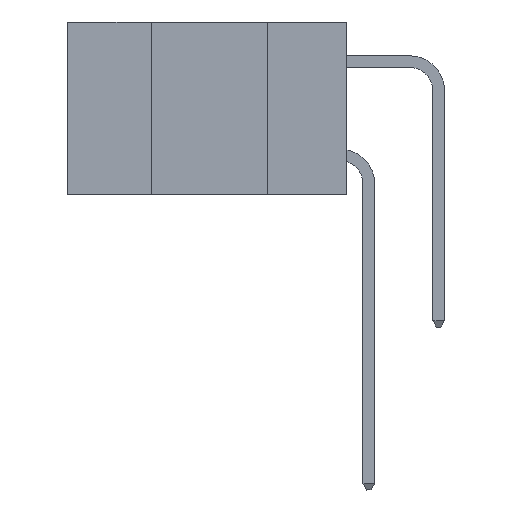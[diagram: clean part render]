
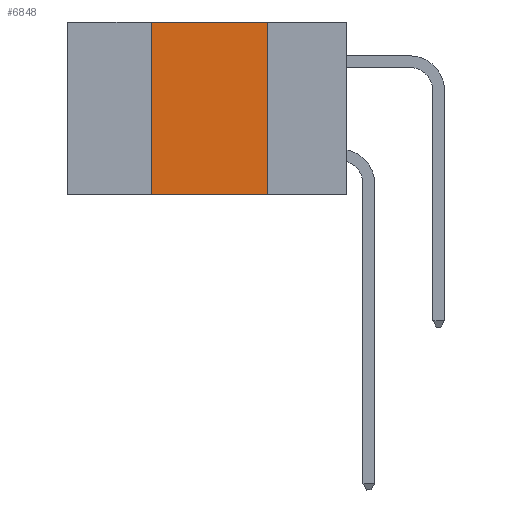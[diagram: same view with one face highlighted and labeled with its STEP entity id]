
A CAD part, left-side view. The second image highlights one B-rep face of the part: STEP entity #6848.
In plain terms, the highlighted planar face has unit normal (-1, 0, 0).
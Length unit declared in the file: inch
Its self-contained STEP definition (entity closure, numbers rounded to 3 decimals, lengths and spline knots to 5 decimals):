
#273 = VECTOR ( 'NONE', #11545, 39.37008 ) ;
#1991 = DIRECTION ( 'NONE',  ( 0., 0., -1. ) ) ;
#3389 = VECTOR ( 'NONE', #14678, 39.37008 ) ;
#4235 = ORIENTED_EDGE ( 'NONE', *, *, #22985, .F. ) ;
#5766 = ORIENTED_EDGE ( 'NONE', *, *, #30835, .F. ) ;
#6083 = LINE ( 'NONE', #36850, #33432 ) ;
#6848 = ADVANCED_FACE ( 'NONE', ( #30297 ), #30507, .F. ) ;
#7326 = CARTESIAN_POINT ( 'NONE',  ( 0., 0.6, -0.37 ) ) ;
#7475 = DIRECTION ( 'NONE',  ( 0., -1., 0. ) ) ;
#7698 = LINE ( 'NONE', #24762, #273 ) ;
#8426 = AXIS2_PLACEMENT_3D ( 'NONE', #30771, #11738, #21469 ) ;
#10468 = ORIENTED_EDGE ( 'NONE', *, *, #29499, .F. ) ;
#11545 = DIRECTION ( 'NONE',  ( 0., -1., 0. ) ) ;
#11738 = DIRECTION ( 'NONE',  ( 1., 0., 0. ) ) ;
#13283 = VERTEX_POINT ( 'NONE', #17419 ) ;
#14207 = LINE ( 'NONE', #7326, #29115 ) ;
#14314 = LINE ( 'NONE', #40411, #3389 ) ;
#14678 = DIRECTION ( 'NONE',  ( 0., 0., 1. ) ) ;
#15131 = EDGE_LOOP ( 'NONE', ( #4235, #5766, #10468, #29826 ) ) ;
#15220 = CARTESIAN_POINT ( 'NONE',  ( 0., 0.17, 0. ) ) ;
#17419 = CARTESIAN_POINT ( 'NONE',  ( 0., 0.17, -0.37 ) ) ;
#20835 = EDGE_CURVE ( 'NONE', #36459, #13283, #14207, .T. ) ;
#21469 = DIRECTION ( 'NONE',  ( 0., 0., -1. ) ) ;
#22985 = EDGE_CURVE ( 'NONE', #38356, #13283, #6083, .T. ) ;
#24762 = CARTESIAN_POINT ( 'NONE',  ( 0., 0.6, 0. ) ) ;
#26040 = VERTEX_POINT ( 'NONE', #34400 ) ;
#29115 = VECTOR ( 'NONE', #7475, 39.37008 ) ;
#29499 = EDGE_CURVE ( 'NONE', #36459, #26040, #14314, .T. ) ;
#29826 = ORIENTED_EDGE ( 'NONE', *, *, #20835, .T. ) ;
#30297 = FACE_OUTER_BOUND ( 'NONE', #15131, .T. ) ;
#30507 = PLANE ( 'NONE',  #8426 ) ;
#30771 = CARTESIAN_POINT ( 'NONE',  ( 0., 0.6, 0. ) ) ;
#30835 = EDGE_CURVE ( 'NONE', #26040, #38356, #7698, .T. ) ;
#33432 = VECTOR ( 'NONE', #1991, 39.37008 ) ;
#34400 = CARTESIAN_POINT ( 'NONE',  ( 0., 0.42, 0. ) ) ;
#36459 = VERTEX_POINT ( 'NONE', #36795 ) ;
#36795 = CARTESIAN_POINT ( 'NONE',  ( 0., 0.42, -0.37 ) ) ;
#36850 = CARTESIAN_POINT ( 'NONE',  ( 0., 0.17, 0. ) ) ;
#38356 = VERTEX_POINT ( 'NONE', #15220 ) ;
#40411 = CARTESIAN_POINT ( 'NONE',  ( 0., 0.42, 0. ) ) ;
